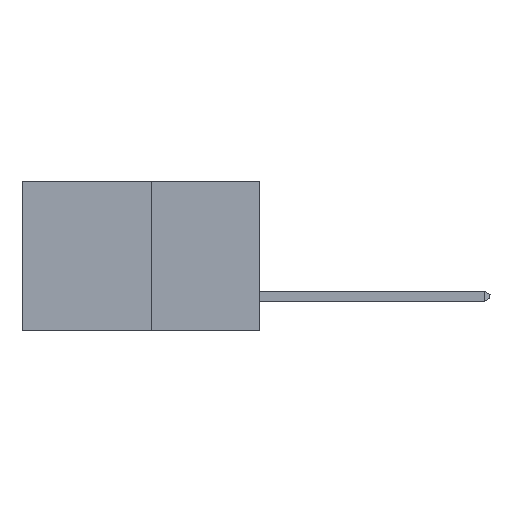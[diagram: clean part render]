
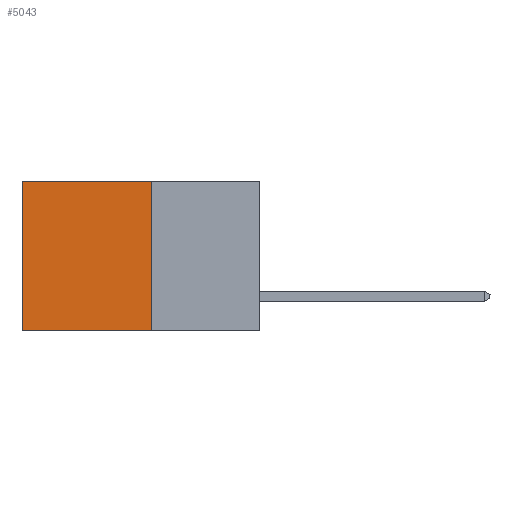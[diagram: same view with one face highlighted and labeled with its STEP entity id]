
A CAD part, left-side view. The second image highlights one B-rep face of the part: STEP entity #5043.
In plain terms, the highlighted planar face has unit normal (-1, 0, 0).
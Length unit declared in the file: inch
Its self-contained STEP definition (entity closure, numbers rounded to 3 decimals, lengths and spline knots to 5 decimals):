
#321 = VERTEX_POINT ( 'NONE', #16251 ) ;
#1903 = VECTOR ( 'NONE', #4741, 39.37008 ) ;
#2121 = CARTESIAN_POINT ( 'NONE',  ( 0.277, 0.27, -0.37 ) ) ;
#2455 = LINE ( 'NONE', #15879, #10489 ) ;
#2989 = EDGE_CURVE ( 'NONE', #8870, #14848, #5690, .T. ) ;
#3253 = ORIENTED_EDGE ( 'NONE', *, *, #15802, .T. ) ;
#3323 = PLANE ( 'NONE',  #16479 ) ;
#4169 = LINE ( 'NONE', #9069, #8398 ) ;
#4741 = DIRECTION ( 'NONE',  ( 0., 0., -1. ) ) ;
#4876 = CARTESIAN_POINT ( 'NONE',  ( 0.277, 0.59, -0.37 ) ) ;
#5043 = ADVANCED_FACE ( 'NONE', ( #9876 ), #3323, .F. ) ;
#5690 = LINE ( 'NONE', #4876, #1903 ) ;
#5891 = EDGE_CURVE ( 'NONE', #7009, #14848, #4169, .T. ) ;
#7009 = VERTEX_POINT ( 'NONE', #15856 ) ;
#7289 = ORIENTED_EDGE ( 'NONE', *, *, #19812, .F. ) ;
#8398 = VECTOR ( 'NONE', #14614, 39.37008 ) ;
#8870 = VERTEX_POINT ( 'NONE', #15025 ) ;
#9069 = CARTESIAN_POINT ( 'NONE',  ( 0.277, 0.27, -0.37 ) ) ;
#9876 = FACE_OUTER_BOUND ( 'NONE', #19279, .T. ) ;
#10489 = VECTOR ( 'NONE', #11267, 39.37008 ) ;
#11267 = DIRECTION ( 'NONE',  ( 0., 1., 0. ) ) ;
#11288 = LINE ( 'NONE', #16288, #18982 ) ;
#12085 = CARTESIAN_POINT ( 'NONE',  ( 0.277, 0.59, -0.37 ) ) ;
#12307 = DIRECTION ( 'NONE',  ( 1., 0., 0. ) ) ;
#13146 = ORIENTED_EDGE ( 'NONE', *, *, #5891, .F. ) ;
#13208 = DIRECTION ( 'NONE',  ( 0., 0., -1. ) ) ;
#14614 = DIRECTION ( 'NONE',  ( 0., 1., 0. ) ) ;
#14848 = VERTEX_POINT ( 'NONE', #12085 ) ;
#15025 = CARTESIAN_POINT ( 'NONE',  ( 0.277, 0.59, 0. ) ) ;
#15802 = EDGE_CURVE ( 'NONE', #321, #8870, #2455, .T. ) ;
#15856 = CARTESIAN_POINT ( 'NONE',  ( 0.277, 0.27, -0.37 ) ) ;
#15879 = CARTESIAN_POINT ( 'NONE',  ( 0.277, 0.27, 0. ) ) ;
#16251 = CARTESIAN_POINT ( 'NONE',  ( 0.277, 0.27, 0. ) ) ;
#16288 = CARTESIAN_POINT ( 'NONE',  ( 0.277, 0.27, -0.37 ) ) ;
#16479 = AXIS2_PLACEMENT_3D ( 'NONE', #2121, #12307, #19042 ) ;
#17071 = ORIENTED_EDGE ( 'NONE', *, *, #2989, .T. ) ;
#18982 = VECTOR ( 'NONE', #13208, 39.37008 ) ;
#19042 = DIRECTION ( 'NONE',  ( 0., 0., -1. ) ) ;
#19279 = EDGE_LOOP ( 'NONE', ( #17071, #13146, #7289, #3253 ) ) ;
#19812 = EDGE_CURVE ( 'NONE', #321, #7009, #11288, .T. ) ;
